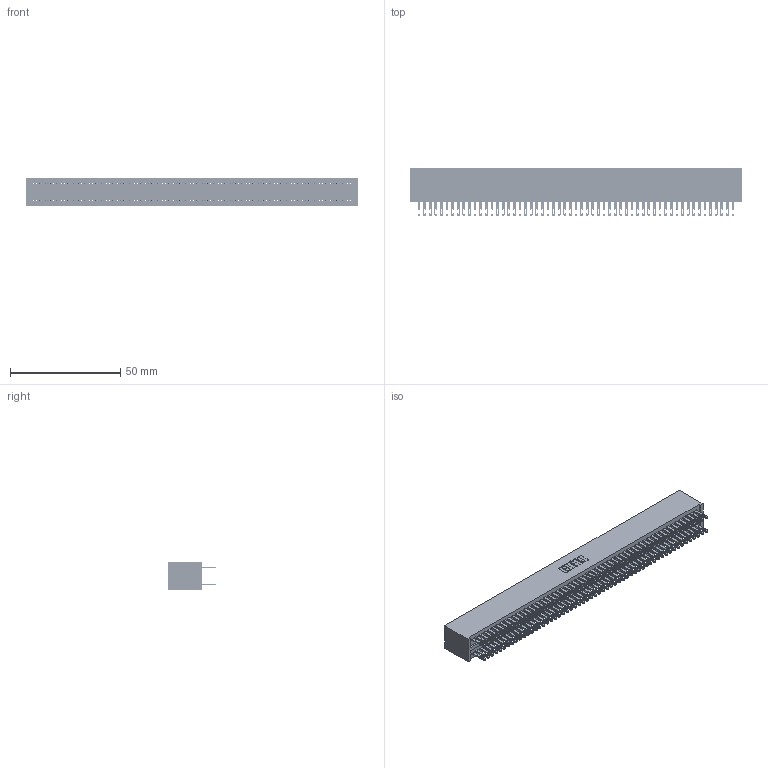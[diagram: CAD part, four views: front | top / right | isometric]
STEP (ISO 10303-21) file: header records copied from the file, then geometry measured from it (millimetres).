
FILE_DESCRIPTION (( 'STEP AP203' ), '1' );
FILE_NAME ('325-114-500-201.STEP', '2020-02-25T07:59:19', ( '' ), ( '' ), 'SwSTEP 2.0', 'SolidWorks 2016', '' );
FILE_SCHEMA (( 'CONFIG_CONTROL_DESIGN' ));
Length unit declared in the file: inch
Products named in the file (3): 325 Part_Lugless; 325-292-001_325-293-100; 325-114-500-201
Assembly tree (115 placements, depth 2):
  325-114-500-201
    325 Part_Lugless
    325-292-001_325-293-100  x114
Bounding box: 150.42 x 21.84 x 12.45 mm (x, y, z)
Volume: 20507.6 mm3; surface area: 27030.4 mm2
Topology: 115 solids, 115 shells, 5578 faces, 17045 edges, 11362 vertices
Faces by surface type: plane 3486, cylinder 2092
Entity records: 34383 total; most frequent: CARTESIAN_POINT 5678, ORIENTED_EDGE 5614, DIRECTION 4819, EDGE_CURVE 2807, LINE 2683, VECTOR 2683, VERTEX_POINT 1870, AXIS2_PLACEMENT_3D 1068
